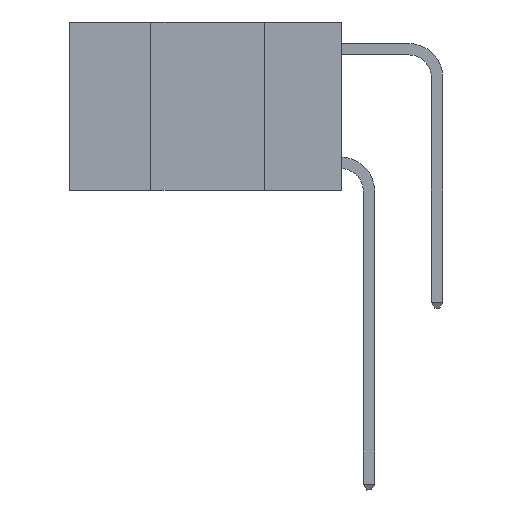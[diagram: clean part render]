
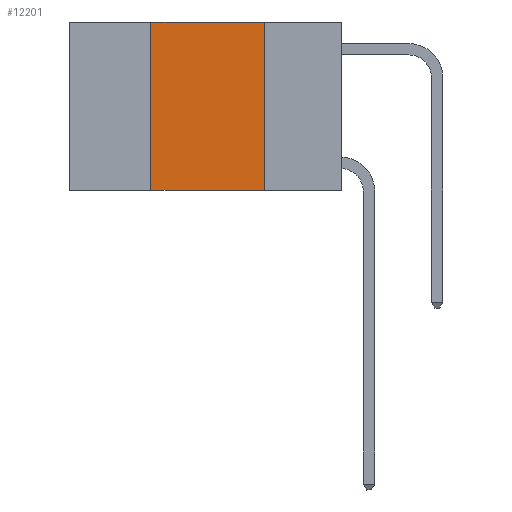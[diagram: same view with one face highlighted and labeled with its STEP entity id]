
A CAD part, left-side view. The second image highlights one B-rep face of the part: STEP entity #12201.
In plain terms, the highlighted planar face has unit normal (-1, 0, 0).
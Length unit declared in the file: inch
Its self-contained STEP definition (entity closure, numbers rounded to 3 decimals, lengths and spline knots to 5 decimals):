
#690 = CARTESIAN_POINT ( 'NONE',  ( 0., 0.42, 0. ) ) ;
#1735 = VERTEX_POINT ( 'NONE', #7986 ) ;
#3200 = LINE ( 'NONE', #11410, #30269 ) ;
#3861 = EDGE_CURVE ( 'NONE', #7909, #25238, #31776, .T. ) ;
#5824 = VECTOR ( 'NONE', #14512, 39.37008 ) ;
#6535 = ORIENTED_EDGE ( 'NONE', *, *, #30078, .F. ) ;
#7246 = VECTOR ( 'NONE', #18892, 39.37008 ) ;
#7909 = VERTEX_POINT ( 'NONE', #14436 ) ;
#7986 = CARTESIAN_POINT ( 'NONE',  ( 0., 0.17, 0. ) ) ;
#8585 = EDGE_CURVE ( 'NONE', #25238, #1735, #32919, .T. ) ;
#10332 = DIRECTION ( 'NONE',  ( 0., 0., -1. ) ) ;
#11410 = CARTESIAN_POINT ( 'NONE',  ( 0., 0.6, -0.37 ) ) ;
#12201 = ADVANCED_FACE ( 'NONE', ( #23567 ), #23013, .F. ) ;
#13046 = EDGE_CURVE ( 'NONE', #7909, #28886, #3200, .T. ) ;
#14436 = CARTESIAN_POINT ( 'NONE',  ( 0., 0.42, -0.37 ) ) ;
#14512 = DIRECTION ( 'NONE',  ( 0., -1., 0. ) ) ;
#15263 = ORIENTED_EDGE ( 'NONE', *, *, #3861, .F. ) ;
#17941 = CARTESIAN_POINT ( 'NONE',  ( 0., 0.6, 0. ) ) ;
#18283 = VECTOR ( 'NONE', #31239, 39.37008 ) ;
#18892 = DIRECTION ( 'NONE',  ( 0., 0., -1. ) ) ;
#21552 = ORIENTED_EDGE ( 'NONE', *, *, #8585, .F. ) ;
#22079 = CARTESIAN_POINT ( 'NONE',  ( 0., 0.6, 0. ) ) ;
#23013 = PLANE ( 'NONE',  #24546 ) ;
#23567 = FACE_OUTER_BOUND ( 'NONE', #27440, .T. ) ;
#24546 = AXIS2_PLACEMENT_3D ( 'NONE', #17941, #25563, #10332 ) ;
#25238 = VERTEX_POINT ( 'NONE', #690 ) ;
#25563 = DIRECTION ( 'NONE',  ( 1., 0., 0. ) ) ;
#26638 = DIRECTION ( 'NONE',  ( 0., -1., 0. ) ) ;
#27440 = EDGE_LOOP ( 'NONE', ( #6535, #21552, #15263, #30386 ) ) ;
#27582 = LINE ( 'NONE', #28975, #7246 ) ;
#28655 = CARTESIAN_POINT ( 'NONE',  ( 0., 0.42, 0. ) ) ;
#28886 = VERTEX_POINT ( 'NONE', #32273 ) ;
#28975 = CARTESIAN_POINT ( 'NONE',  ( 0., 0.17, 0. ) ) ;
#30078 = EDGE_CURVE ( 'NONE', #1735, #28886, #27582, .T. ) ;
#30269 = VECTOR ( 'NONE', #26638, 39.37008 ) ;
#30386 = ORIENTED_EDGE ( 'NONE', *, *, #13046, .T. ) ;
#31239 = DIRECTION ( 'NONE',  ( 0., 0., 1. ) ) ;
#31776 = LINE ( 'NONE', #28655, #18283 ) ;
#32273 = CARTESIAN_POINT ( 'NONE',  ( 0., 0.17, -0.37 ) ) ;
#32919 = LINE ( 'NONE', #22079, #5824 ) ;
